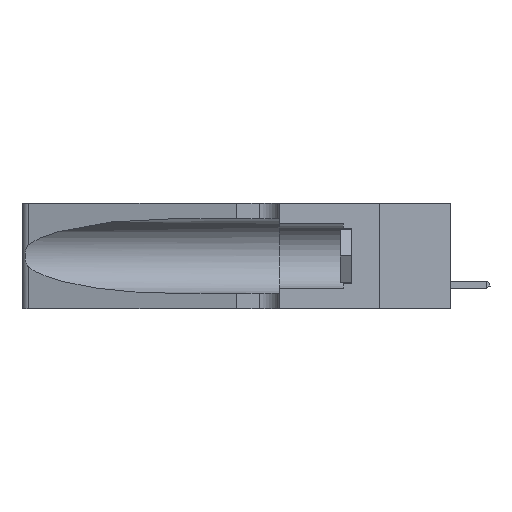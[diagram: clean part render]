
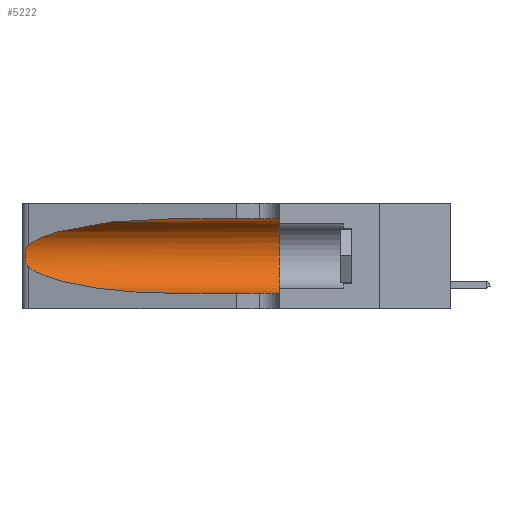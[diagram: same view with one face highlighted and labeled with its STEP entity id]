
A CAD part, left-side view. The second image highlights one B-rep face of the part: STEP entity #5222.
In plain terms, the highlighted cylindrical face has radius 3.308 mm (diameter 6.617 mm), a partial arc.
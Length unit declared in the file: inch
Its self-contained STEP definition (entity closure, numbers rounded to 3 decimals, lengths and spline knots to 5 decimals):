
#218 = CARTESIAN_POINT ( 'NONE',  ( 0.25487, 1.22718, 0.14631 ) ) ;
#822 = CARTESIAN_POINT ( 'NONE',  ( 0.18966, 0.96281, 0.05475 ) ) ;
#1062 = AXIS2_PLACEMENT_3D ( 'NONE', #16480, #8403, #3894 ) ;
#1535 = CYLINDRICAL_SURFACE ( 'NONE', #17364, 0.13025 ) ;
#1572 = EDGE_CURVE ( 'NONE', #11505, #4441, #4003, .T. ) ;
#1876 = CARTESIAN_POINT ( 'NONE',  ( 0.25639, 1.23186, 0.15144 ) ) ;
#2228 = CARTESIAN_POINT ( 'NONE',  ( 0.1305, 0.72297, 0.05475 ) ) ;
#2330 = ORIENTED_EDGE ( 'NONE', *, *, #1572, .F. ) ;
#2683 = CARTESIAN_POINT ( 'NONE',  ( 0.25487, 1.22718, 0.14631 ) ) ;
#3061 = EDGE_CURVE ( 'NONE', #11505, #11163, #4825, .T. ) ;
#3402 = DIRECTION ( 'NONE',  ( 0., -1., 0. ) ) ;
#3468 = ORIENTED_EDGE ( 'NONE', *, *, #3061, .T. ) ;
#3742 = CARTESIAN_POINT ( 'NONE',  ( 0.1305, 0.72297, 0.31525 ) ) ;
#3894 = DIRECTION ( 'NONE',  ( 0., 0., 1. ) ) ;
#4003 = LINE ( 'NONE', #11660, #16489 ) ;
#4441 = VERTEX_POINT ( 'NONE', #9143 ) ;
#4787 = CARTESIAN_POINT ( 'NONE',  ( 0.25787, 1.23484, 0.2124 ) ) ;
#4788 = CARTESIAN_POINT ( 'NONE',  ( 0.1305, 0.72297, 0.31525 ) ) ;
#4825 =( BOUNDED_CURVE ( )  B_SPLINE_CURVE ( 3, ( #3742, #18653, #15726, #17322 ),
 .UNSPECIFIED., .F., .T. ) 
 B_SPLINE_CURVE_WITH_KNOTS ( ( 4, 4 ),
 ( 1.5708, 2.84003 ),
 .UNSPECIFIED. ) 
 CURVE ( )  GEOMETRIC_REPRESENTATION_ITEM ( )  RATIONAL_B_SPLINE_CURVE ( ( 1., 0.87, 0.87, 1. ) ) 
 REPRESENTATION_ITEM ( '' )  );
#4841 = DIRECTION ( 'NONE',  ( 0., 0., -1. ) ) ;
#4860 = CARTESIAN_POINT ( 'NONE',  ( 0.26017, 1.23833, 0.17102 ) ) ;
#5222 = ADVANCED_FACE ( 'NONE', ( #18067 ), #1535, .F. ) ;
#6305 = CARTESIAN_POINT ( 'NONE',  ( 0.26075, 1.23896, 0.19203 ) ) ;
#7770 = CARTESIAN_POINT ( 'NONE',  ( 0.25789, 1.23486, 0.15765 ) ) ;
#8403 = DIRECTION ( 'NONE',  ( 0., 1., 0. ) ) ;
#8511 = CARTESIAN_POINT ( 'NONE',  ( 0.25487, 1.22718, 0.14631 ) ) ;
#8801 = LINE ( 'NONE', #17130, #13495 ) ;
#9043 = CARTESIAN_POINT ( 'NONE',  ( 0.25555, 1.22994, 0.2215 ) ) ;
#9136 = ORIENTED_EDGE ( 'NONE', *, *, #13399, .F. ) ;
#9143 = CARTESIAN_POINT ( 'NONE',  ( 0.1305, 0.35, 0.31525 ) ) ;
#9219 = B_SPLINE_CURVE_WITH_KNOTS ( 'NONE', 3,
 ( #16666, #9043, #19581, #4787, #12272, #13891, #6305, #18523, #4860, #9509, #7770, #1876, #15395, #218 ),
 .UNSPECIFIED., .F., .F.,
 ( 4, 2, 2, 2, 2, 2, 4 ),
 ( 0., 0.00027, 0.00053, 0.00107, 0.0016, 0.00187, 0.00214 ),
 .UNSPECIFIED. ) ;
#9248 = VERTEX_POINT ( 'NONE', #16403 ) ;
#9509 = CARTESIAN_POINT ( 'NONE',  ( 0.25856, 1.23593, 0.16098 ) ) ;
#9516 = EDGE_CURVE ( 'NONE', #15662, #14449, #17149, .T. ) ;
#9929 = CARTESIAN_POINT ( 'NONE',  ( 0.2373, 1.15595, 0.08982 ) ) ;
#11163 = VERTEX_POINT ( 'NONE', #16259 ) ;
#11505 = VERTEX_POINT ( 'NONE', #4788 ) ;
#11556 = EDGE_LOOP ( 'NONE', ( #3468, #17600, #18900, #18599, #9136, #2330 ) ) ;
#11660 = CARTESIAN_POINT ( 'NONE',  ( 0.1305, 1.61858, 0.31525 ) ) ;
#11870 = EDGE_CURVE ( 'NONE', #11163, #15662, #9219, .T. ) ;
#12272 = CARTESIAN_POINT ( 'NONE',  ( 0.25854, 1.2359, 0.20912 ) ) ;
#13399 = EDGE_CURVE ( 'NONE', #4441, #9248, #14049, .T. ) ;
#13495 = VECTOR ( 'NONE', #3402, 39.37008 ) ;
#13878 = CARTESIAN_POINT ( 'NONE',  ( 0.1305, 1.61858, 0.185 ) ) ;
#13891 = CARTESIAN_POINT ( 'NONE',  ( 0.26018, 1.23835, 0.19895 ) ) ;
#14049 = CIRCLE ( 'NONE', #1062, 0.13025 ) ;
#14449 = VERTEX_POINT ( 'NONE', #2228 ) ;
#15395 = CARTESIAN_POINT ( 'NONE',  ( 0.25555, 1.22993, 0.14849 ) ) ;
#15445 = DIRECTION ( 'NONE',  ( 0., -1., 0. ) ) ;
#15662 = VERTEX_POINT ( 'NONE', #2683 ) ;
#15726 = CARTESIAN_POINT ( 'NONE',  ( 0.2373, 1.15595, 0.28018 ) ) ;
#15944 = CARTESIAN_POINT ( 'NONE',  ( 0.1305, 0.72297, 0.05475 ) ) ;
#16259 = CARTESIAN_POINT ( 'NONE',  ( 0.25487, 1.22718, 0.22369 ) ) ;
#16397 = DIRECTION ( 'NONE',  ( 0., -1., 0. ) ) ;
#16403 = CARTESIAN_POINT ( 'NONE',  ( 0.1305, 0.35, 0.05475 ) ) ;
#16480 = CARTESIAN_POINT ( 'NONE',  ( 0.1305, 0.35, 0.185 ) ) ;
#16489 = VECTOR ( 'NONE', #16397, 39.37008 ) ;
#16666 = CARTESIAN_POINT ( 'NONE',  ( 0.25487, 1.22718, 0.22369 ) ) ;
#17130 = CARTESIAN_POINT ( 'NONE',  ( 0.1305, 1.61858, 0.05475 ) ) ;
#17149 =( BOUNDED_CURVE ( )  B_SPLINE_CURVE ( 3, ( #8511, #9929, #822, #15944 ),
 .UNSPECIFIED., .F., .T. ) 
 B_SPLINE_CURVE_WITH_KNOTS ( ( 4, 4 ),
 ( 3.44316, 4.71239 ),
 .UNSPECIFIED. ) 
 CURVE ( )  GEOMETRIC_REPRESENTATION_ITEM ( )  RATIONAL_B_SPLINE_CURVE ( ( 1., 0.87, 0.87, 1. ) ) 
 REPRESENTATION_ITEM ( '' )  );
#17322 = CARTESIAN_POINT ( 'NONE',  ( 0.25487, 1.22718, 0.22369 ) ) ;
#17364 = AXIS2_PLACEMENT_3D ( 'NONE', #13878, #15445, #4841 ) ;
#17600 = ORIENTED_EDGE ( 'NONE', *, *, #11870, .T. ) ;
#18067 = FACE_OUTER_BOUND ( 'NONE', #11556, .T. ) ;
#18523 = CARTESIAN_POINT ( 'NONE',  ( 0.26075, 1.23896, 0.178 ) ) ;
#18599 = ORIENTED_EDGE ( 'NONE', *, *, #18626, .T. ) ;
#18626 = EDGE_CURVE ( 'NONE', #14449, #9248, #8801, .T. ) ;
#18653 = CARTESIAN_POINT ( 'NONE',  ( 0.18966, 0.96281, 0.31525 ) ) ;
#18900 = ORIENTED_EDGE ( 'NONE', *, *, #9516, .T. ) ;
#19581 = CARTESIAN_POINT ( 'NONE',  ( 0.25639, 1.23184, 0.21858 ) ) ;
